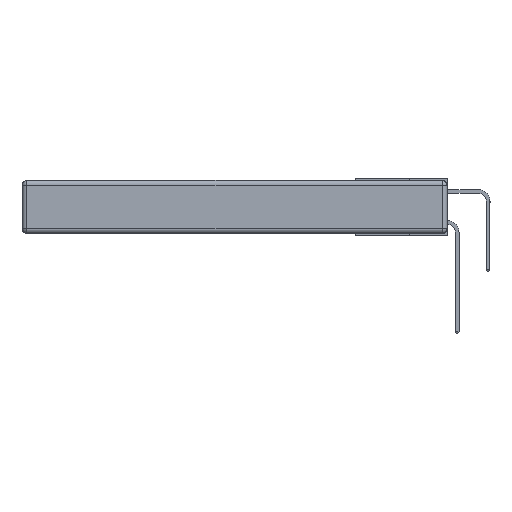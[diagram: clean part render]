
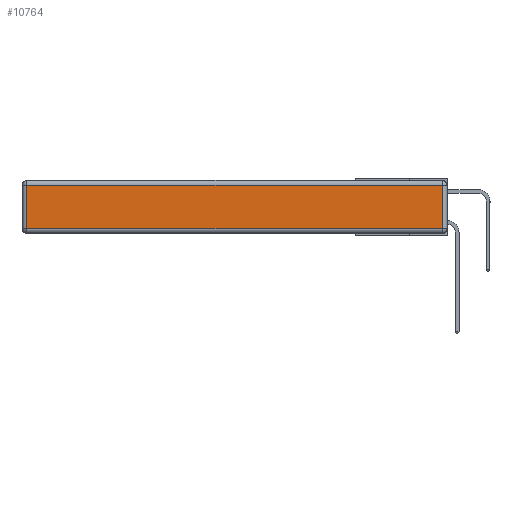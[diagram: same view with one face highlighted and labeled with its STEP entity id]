
A CAD part, left-side view. The second image highlights one B-rep face of the part: STEP entity #10764.
In plain terms, the highlighted planar face has unit normal (-1, 0, 0).
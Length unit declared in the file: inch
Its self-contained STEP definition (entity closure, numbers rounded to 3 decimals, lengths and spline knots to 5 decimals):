
#431 = DIRECTION ( 'NONE',  ( 0., 1., 0. ) ) ;
#746 = ORIENTED_EDGE ( 'NONE', *, *, #13639, .T. ) ;
#2056 = VECTOR ( 'NONE', #15291, 39.37008 ) ;
#2164 = VECTOR ( 'NONE', #14890, 39.37008 ) ;
#2650 = VECTOR ( 'NONE', #431, 39.37008 ) ;
#2659 = CARTESIAN_POINT ( 'NONE',  ( 0., 2.72, -0.343 ) ) ;
#2661 = ORIENTED_EDGE ( 'NONE', *, *, #15560, .T. ) ;
#3427 = CARTESIAN_POINT ( 'NONE',  ( 0., 0., -0.343 ) ) ;
#4997 = LINE ( 'NONE', #18433, #2650 ) ;
#7062 = LINE ( 'NONE', #14286, #19581 ) ;
#7180 = LINE ( 'NONE', #2659, #2056 ) ;
#9213 = EDGE_CURVE ( 'NONE', #32441, #18052, #7062, .T. ) ;
#9858 = CARTESIAN_POINT ( 'NONE',  ( 0., 2.72, -0.03 ) ) ;
#10197 = VERTEX_POINT ( 'NONE', #9858 ) ;
#10764 = ADVANCED_FACE ( 'NONE', ( #28971 ), #31291, .T. ) ;
#11334 = DIRECTION ( 'NONE',  ( 0., 0., 1. ) ) ;
#13639 = EDGE_CURVE ( 'NONE', #18052, #26953, #16717, .T. ) ;
#14247 = CARTESIAN_POINT ( 'NONE',  ( 0., 0.03, -0.03 ) ) ;
#14286 = CARTESIAN_POINT ( 'NONE',  ( 0., 0., -0.313 ) ) ;
#14890 = DIRECTION ( 'NONE',  ( 0., 0., 1. ) ) ;
#15291 = DIRECTION ( 'NONE',  ( 0., 0., -1. ) ) ;
#15560 = EDGE_CURVE ( 'NONE', #10197, #32441, #7180, .T. ) ;
#16717 = LINE ( 'NONE', #25324, #2164 ) ;
#17719 = ORIENTED_EDGE ( 'NONE', *, *, #28511, .T. ) ;
#18052 = VERTEX_POINT ( 'NONE', #22223 ) ;
#18433 = CARTESIAN_POINT ( 'NONE',  ( 0., 2.75, -0.03 ) ) ;
#18695 = CARTESIAN_POINT ( 'NONE',  ( 0., 2.72, -0.313 ) ) ;
#19581 = VECTOR ( 'NONE', #24115, 39.37008 ) ;
#22223 = CARTESIAN_POINT ( 'NONE',  ( 0., 0.03, -0.313 ) ) ;
#24115 = DIRECTION ( 'NONE',  ( 0., -1., 0. ) ) ;
#25324 = CARTESIAN_POINT ( 'NONE',  ( 0., 0.03, -0.343 ) ) ;
#26193 = DIRECTION ( 'NONE',  ( -1., 0., 0. ) ) ;
#26933 = EDGE_LOOP ( 'NONE', ( #29046, #746, #17719, #2661 ) ) ;
#26953 = VERTEX_POINT ( 'NONE', #14247 ) ;
#28511 = EDGE_CURVE ( 'NONE', #26953, #10197, #4997, .T. ) ;
#28971 = FACE_OUTER_BOUND ( 'NONE', #26933, .T. ) ;
#29046 = ORIENTED_EDGE ( 'NONE', *, *, #9213, .T. ) ;
#29698 = AXIS2_PLACEMENT_3D ( 'NONE', #3427, #26193, #11334 ) ;
#31291 = PLANE ( 'NONE',  #29698 ) ;
#32441 = VERTEX_POINT ( 'NONE', #18695 ) ;
